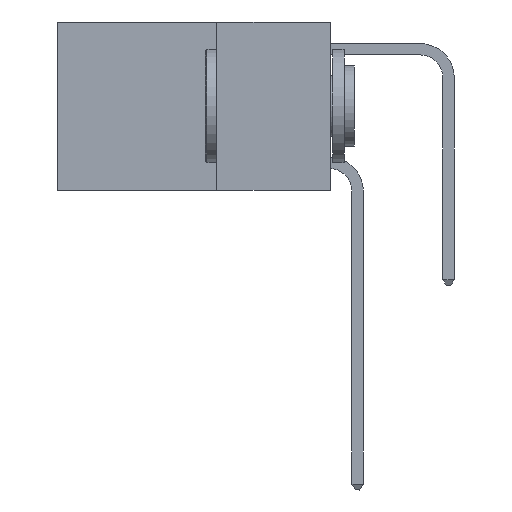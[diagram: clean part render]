
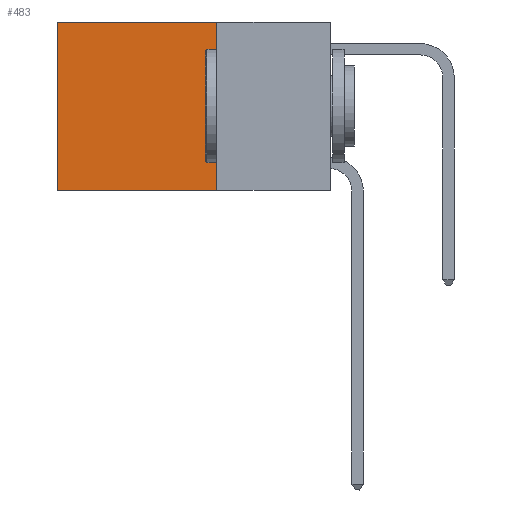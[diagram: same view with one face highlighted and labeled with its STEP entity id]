
A CAD part, left-side view. The second image highlights one B-rep face of the part: STEP entity #483.
In plain terms, the highlighted planar face has unit normal (-1, 0, 0).
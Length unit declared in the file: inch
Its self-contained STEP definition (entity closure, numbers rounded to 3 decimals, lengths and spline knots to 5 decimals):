
#86 = EDGE_CURVE ( 'NONE', #2062, #14025, #9761, .T. ) ;
#208 = VECTOR ( 'NONE', #6771, 39.37008 ) ;
#483 = ADVANCED_FACE ( 'NONE', ( #3304 ), #788, .F. ) ;
#788 = PLANE ( 'NONE',  #6507 ) ;
#1269 = CARTESIAN_POINT ( 'NONE',  ( 0.2625, 0.6, 0. ) ) ;
#1350 = VERTEX_POINT ( 'NONE', #2630 ) ;
#1872 = VECTOR ( 'NONE', #2604, 39.37008 ) ;
#2062 = VERTEX_POINT ( 'NONE', #1269 ) ;
#2604 = DIRECTION ( 'NONE',  ( 0., 0., -1. ) ) ;
#2630 = CARTESIAN_POINT ( 'NONE',  ( 0.2625, 0.25, 0. ) ) ;
#3304 = FACE_OUTER_BOUND ( 'NONE', #15716, .T. ) ;
#3310 = ORIENTED_EDGE ( 'NONE', *, *, #13351, .T. ) ;
#3362 = ORIENTED_EDGE ( 'NONE', *, *, #7287, .F. ) ;
#3783 = ORIENTED_EDGE ( 'NONE', *, *, #86, .T. ) ;
#3878 = DIRECTION ( 'NONE',  ( 1., 0., 0. ) ) ;
#4480 = CARTESIAN_POINT ( 'NONE',  ( 0.2625, 0.6, -0.37 ) ) ;
#5370 = CARTESIAN_POINT ( 'NONE',  ( 0.2625, 0.25, -0.37 ) ) ;
#6090 = VECTOR ( 'NONE', #7319, 39.37008 ) ;
#6507 = AXIS2_PLACEMENT_3D ( 'NONE', #8239, #3878, #14086 ) ;
#6771 = DIRECTION ( 'NONE',  ( 0., 1., 0. ) ) ;
#7287 = EDGE_CURVE ( 'NONE', #1350, #14420, #9969, .T. ) ;
#7319 = DIRECTION ( 'NONE',  ( 0., 0., -1. ) ) ;
#8239 = CARTESIAN_POINT ( 'NONE',  ( 0.2625, 0.25, 0. ) ) ;
#9761 = LINE ( 'NONE', #14290, #1872 ) ;
#9969 = LINE ( 'NONE', #17494, #6090 ) ;
#10467 = CARTESIAN_POINT ( 'NONE',  ( 0.2625, 0.25, 0. ) ) ;
#10531 = DIRECTION ( 'NONE',  ( 0., 1., 0. ) ) ;
#10636 = LINE ( 'NONE', #10467, #17851 ) ;
#11608 = LINE ( 'NONE', #14076, #208 ) ;
#12418 = EDGE_CURVE ( 'NONE', #14420, #14025, #11608, .T. ) ;
#13351 = EDGE_CURVE ( 'NONE', #1350, #2062, #10636, .T. ) ;
#14025 = VERTEX_POINT ( 'NONE', #4480 ) ;
#14076 = CARTESIAN_POINT ( 'NONE',  ( 0.2625, 0.25, -0.37 ) ) ;
#14086 = DIRECTION ( 'NONE',  ( 0., 0., -1. ) ) ;
#14290 = CARTESIAN_POINT ( 'NONE',  ( 0.2625, 0.6, 0. ) ) ;
#14420 = VERTEX_POINT ( 'NONE', #5370 ) ;
#15716 = EDGE_LOOP ( 'NONE', ( #3783, #16114, #3362, #3310 ) ) ;
#16114 = ORIENTED_EDGE ( 'NONE', *, *, #12418, .F. ) ;
#17494 = CARTESIAN_POINT ( 'NONE',  ( 0.2625, 0.25, 0. ) ) ;
#17851 = VECTOR ( 'NONE', #10531, 39.37008 ) ;
